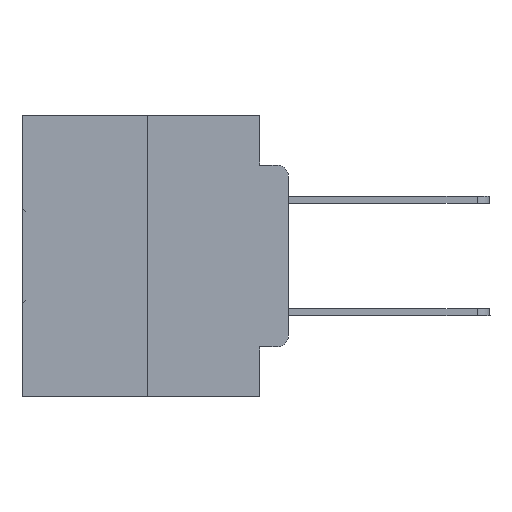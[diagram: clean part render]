
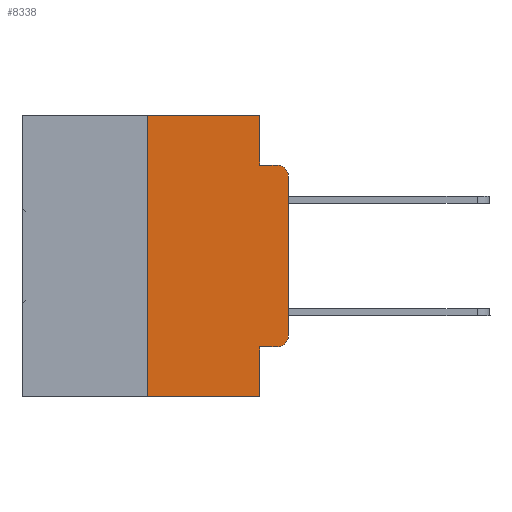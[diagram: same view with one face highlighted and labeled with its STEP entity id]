
A CAD part, left-side view. The second image highlights one B-rep face of the part: STEP entity #8338.
In plain terms, the highlighted planar face has unit normal (-1, 0, 0).
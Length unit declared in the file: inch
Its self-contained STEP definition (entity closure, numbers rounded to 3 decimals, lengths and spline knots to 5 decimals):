
#294 = CARTESIAN_POINT ( 'NONE',  ( 0., 0., 0. ) ) ;
#408 = DIRECTION ( 'NONE',  ( 0., 0., 1. ) ) ;
#553 = VECTOR ( 'NONE', #7604, 39.37008 ) ;
#746 = VERTEX_POINT ( 'NONE', #14433 ) ;
#898 = LINE ( 'NONE', #16350, #9857 ) ;
#1179 = CARTESIAN_POINT ( 'NONE',  ( 0., 0.051, -0.5 ) ) ;
#1525 = LINE ( 'NONE', #7873, #9198 ) ;
#3037 = VECTOR ( 'NONE', #19244, 39.37008 ) ;
#3281 = VERTEX_POINT ( 'NONE', #19794 ) ;
#3328 = CARTESIAN_POINT ( 'NONE',  ( 0., 0.02, -0.0885 ) ) ;
#3724 = CARTESIAN_POINT ( 'NONE',  ( 0., 0.051, 0. ) ) ;
#4080 = EDGE_CURVE ( 'NONE', #27750, #7078, #898, .T. ) ;
#4211 = CARTESIAN_POINT ( 'NONE',  ( 0., 0.051, -0.4115 ) ) ;
#4474 = CARTESIAN_POINT ( 'NONE',  ( 0., 0.473, 0. ) ) ;
#5251 = EDGE_CURVE ( 'NONE', #26541, #27750, #11774, .T. ) ;
#5499 = DIRECTION ( 'NONE',  ( -1., 0., 0. ) ) ;
#6703 = LINE ( 'NONE', #4211, #19262 ) ;
#6748 = FACE_OUTER_BOUND ( 'NONE', #9018, .T. ) ;
#7078 = VERTEX_POINT ( 'NONE', #25295 ) ;
#7205 = DIRECTION ( 'NONE',  ( 0., 0., -1. ) ) ;
#7217 = LINE ( 'NONE', #23656, #20208 ) ;
#7604 = DIRECTION ( 'NONE',  ( 0., 0., -1. ) ) ;
#7806 = CARTESIAN_POINT ( 'NONE',  ( 0., 0.02, -0.3915 ) ) ;
#7873 = CARTESIAN_POINT ( 'NONE',  ( 0., 0.051, -0.0885 ) ) ;
#8338 = ADVANCED_FACE ( 'NONE', ( #6748 ), #14756, .F. ) ;
#8664 = VECTOR ( 'NONE', #408, 39.37008 ) ;
#9018 = EDGE_LOOP ( 'NONE', ( #30513, #24454, #13274, #18710, #14215, #24085, #22571, #11426, #26038, #26083 ) ) ;
#9198 = VECTOR ( 'NONE', #17860, 39.37008 ) ;
#9857 = VECTOR ( 'NONE', #29607, 39.37008 ) ;
#10075 = DIRECTION ( 'NONE',  ( 0., 0., 1. ) ) ;
#10337 = LINE ( 'NONE', #3724, #3037 ) ;
#10351 = EDGE_CURVE ( 'NONE', #20480, #15330, #10337, .T. ) ;
#10500 = EDGE_CURVE ( 'NONE', #20480, #13692, #6703, .T. ) ;
#11231 = EDGE_CURVE ( 'NONE', #20633, #3281, #29308, .T. ) ;
#11426 = ORIENTED_EDGE ( 'NONE', *, *, #10351, .F. ) ;
#11774 = LINE ( 'NONE', #20512, #29992 ) ;
#11785 = DIRECTION ( 'NONE',  ( 0., -1., 0. ) ) ;
#13136 = DIRECTION ( 'NONE',  ( 0., -1., 0. ) ) ;
#13265 = CARTESIAN_POINT ( 'NONE',  ( 0., 0.051, -0.4115 ) ) ;
#13274 = ORIENTED_EDGE ( 'NONE', *, *, #19656, .F. ) ;
#13692 = VERTEX_POINT ( 'NONE', #18235 ) ;
#14215 = ORIENTED_EDGE ( 'NONE', *, *, #4080, .F. ) ;
#14433 = CARTESIAN_POINT ( 'NONE',  ( 0., 0.051, -0.0885 ) ) ;
#14756 = PLANE ( 'NONE',  #22852 ) ;
#14857 = CIRCLE ( 'NONE', #28715, 0.02 ) ;
#15330 = VERTEX_POINT ( 'NONE', #1179 ) ;
#16350 = CARTESIAN_POINT ( 'NONE',  ( 0., 0.473, 0. ) ) ;
#17860 = DIRECTION ( 'NONE',  ( 0., -1., 0. ) ) ;
#17993 = LINE ( 'NONE', #20537, #553 ) ;
#18235 = CARTESIAN_POINT ( 'NONE',  ( 0., 0.02, -0.4115 ) ) ;
#18710 = ORIENTED_EDGE ( 'NONE', *, *, #23232, .F. ) ;
#19244 = DIRECTION ( 'NONE',  ( 0., 0., -1. ) ) ;
#19262 = VECTOR ( 'NONE', #11785, 39.37008 ) ;
#19656 = EDGE_CURVE ( 'NONE', #746, #33290, #1525, .T. ) ;
#19794 = CARTESIAN_POINT ( 'NONE',  ( 0., 0., -0.1085 ) ) ;
#20208 = VECTOR ( 'NONE', #13136, 39.37008 ) ;
#20480 = VERTEX_POINT ( 'NONE', #13265 ) ;
#20512 = CARTESIAN_POINT ( 'NONE',  ( 0., 0.25, 0. ) ) ;
#20537 = CARTESIAN_POINT ( 'NONE',  ( 0., 0.051, 0. ) ) ;
#20633 = VERTEX_POINT ( 'NONE', #21415 ) ;
#21088 = EDGE_CURVE ( 'NONE', #13692, #20633, #14857, .T. ) ;
#21415 = CARTESIAN_POINT ( 'NONE',  ( 0., 0., -0.3915 ) ) ;
#21469 = EDGE_CURVE ( 'NONE', #3281, #33290, #30987, .T. ) ;
#22260 = AXIS2_PLACEMENT_3D ( 'NONE', #30178, #24999, #7205 ) ;
#22466 = DIRECTION ( 'NONE',  ( 1., 0., 0. ) ) ;
#22571 = ORIENTED_EDGE ( 'NONE', *, *, #26767, .T. ) ;
#22585 = DIRECTION ( 'NONE',  ( 0., 0., -1. ) ) ;
#22852 = AXIS2_PLACEMENT_3D ( 'NONE', #4474, #22466, #22585 ) ;
#23232 = EDGE_CURVE ( 'NONE', #7078, #746, #17993, .T. ) ;
#23656 = CARTESIAN_POINT ( 'NONE',  ( 0., 0.473, -0.5 ) ) ;
#24085 = ORIENTED_EDGE ( 'NONE', *, *, #5251, .F. ) ;
#24222 = CARTESIAN_POINT ( 'NONE',  ( 0., 0.25, 0. ) ) ;
#24454 = ORIENTED_EDGE ( 'NONE', *, *, #21469, .T. ) ;
#24999 = DIRECTION ( 'NONE',  ( -1., 0., 0. ) ) ;
#25295 = CARTESIAN_POINT ( 'NONE',  ( 0., 0.051, 0. ) ) ;
#26038 = ORIENTED_EDGE ( 'NONE', *, *, #10500, .T. ) ;
#26083 = ORIENTED_EDGE ( 'NONE', *, *, #21088, .T. ) ;
#26541 = VERTEX_POINT ( 'NONE', #28113 ) ;
#26767 = EDGE_CURVE ( 'NONE', #26541, #15330, #7217, .T. ) ;
#27750 = VERTEX_POINT ( 'NONE', #24222 ) ;
#28113 = CARTESIAN_POINT ( 'NONE',  ( 0., 0.25, -0.5 ) ) ;
#28715 = AXIS2_PLACEMENT_3D ( 'NONE', #7806, #5499, #30976 ) ;
#29308 = LINE ( 'NONE', #294, #8664 ) ;
#29607 = DIRECTION ( 'NONE',  ( 0., -1., 0. ) ) ;
#29992 = VECTOR ( 'NONE', #10075, 39.37008 ) ;
#30178 = CARTESIAN_POINT ( 'NONE',  ( 0., 0.02, -0.1085 ) ) ;
#30513 = ORIENTED_EDGE ( 'NONE', *, *, #11231, .T. ) ;
#30976 = DIRECTION ( 'NONE',  ( 0., 0., -1. ) ) ;
#30987 = CIRCLE ( 'NONE', #22260, 0.02 ) ;
#33290 = VERTEX_POINT ( 'NONE', #3328 ) ;
